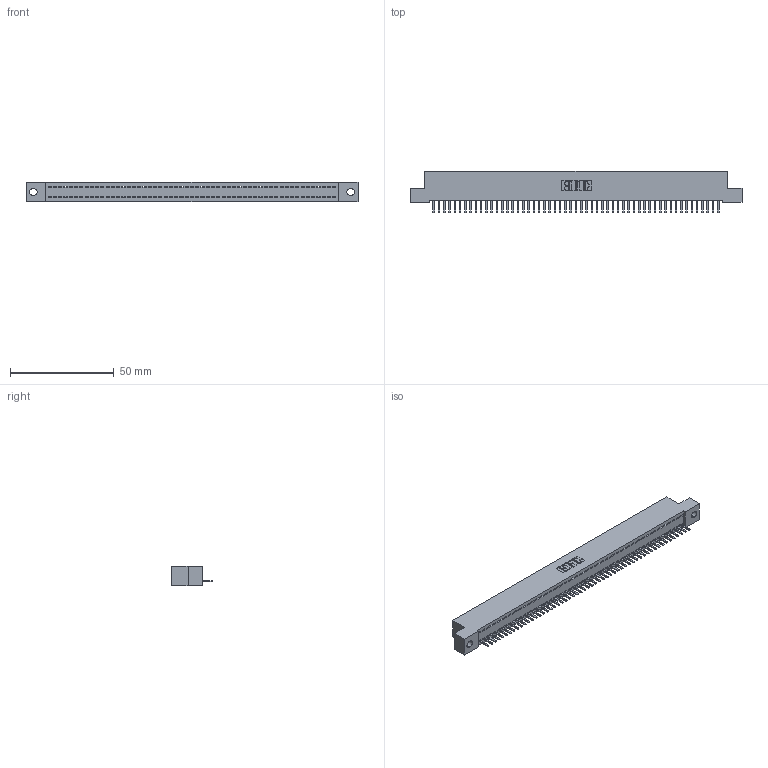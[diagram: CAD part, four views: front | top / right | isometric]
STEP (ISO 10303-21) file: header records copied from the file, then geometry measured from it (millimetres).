
FILE_DESCRIPTION (( 'STEP AP203' ), '1' );
FILE_NAME ('342-055-520-102.STEP', '2018-08-13T01:15:56', ( '' ), ( '' ), 'SwSTEP 2.0', 'SolidWorks 2016', '' );
FILE_SCHEMA (( 'CONFIG_CONTROL_DESIGN' ));
Length unit declared in the file: inch
Products named in the file (3): 342 Part_.128 Slot; 345-292-001_345-293-120; 342-055-520-102
Assembly tree (56 placements, depth 2):
  342-055-520-102
    342 Part_.128 Slot
    345-292-001_345-293-120  x55
Bounding box: 160.02 x 20.02 x 9.4 mm (x, y, z)
Volume: 13868.1 mm3; surface area: 19861 mm2
Topology: 56 solids, 56 shells, 3524 faces, 10431 edges, 6806 vertices
Faces by surface type: plane 2490, cylinder 1034
Entity records: 32059 total; most frequent: CARTESIAN_POINT 5547, ORIENTED_EDGE 5526, DIRECTION 4641, EDGE_CURVE 2763, LINE 2631, VECTOR 2631, VERTEX_POINT 1838, AXIS2_PLACEMENT_3D 1005
